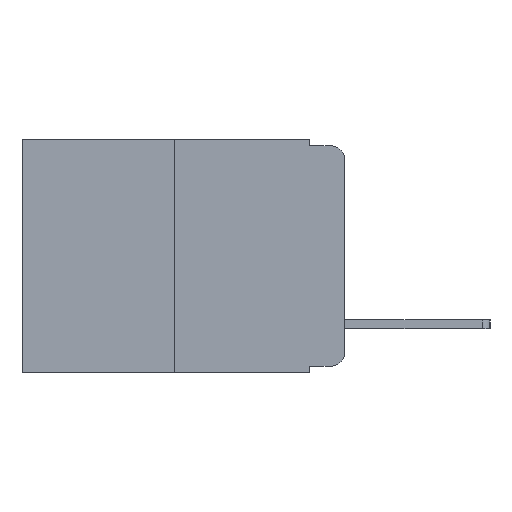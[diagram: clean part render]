
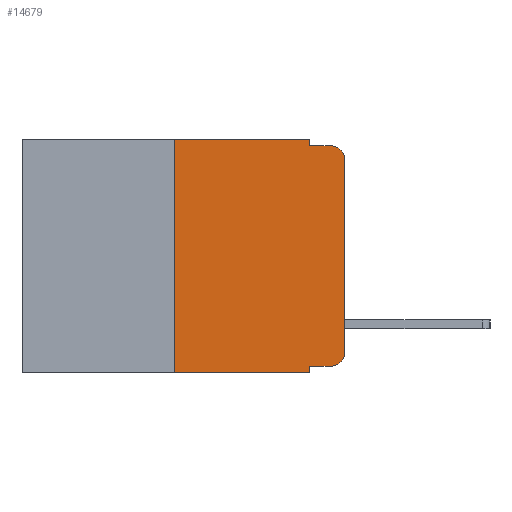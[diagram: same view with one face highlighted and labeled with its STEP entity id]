
A CAD part, left-side view. The second image highlights one B-rep face of the part: STEP entity #14679.
In plain terms, the highlighted planar face has unit normal (-1, 0, 0).
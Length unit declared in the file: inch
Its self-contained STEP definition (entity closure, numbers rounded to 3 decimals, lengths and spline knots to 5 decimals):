
#85 = EDGE_CURVE ( 'NONE', #4995, #4182, #15944, .T. ) ;
#352 = CARTESIAN_POINT ( 'NONE',  ( 0., 0.25, 0. ) ) ;
#551 = VERTEX_POINT ( 'NONE', #2839 ) ;
#724 = CARTESIAN_POINT ( 'NONE',  ( 0., 0., 0. ) ) ;
#828 = EDGE_CURVE ( 'NONE', #551, #3973, #16782, .T. ) ;
#1203 = CARTESIAN_POINT ( 'NONE',  ( 0., 0.02, -0.03 ) ) ;
#1245 = EDGE_CURVE ( 'NONE', #3353, #13988, #9838, .T. ) ;
#1273 = ORIENTED_EDGE ( 'NONE', *, *, #11226, .F. ) ;
#1449 = ORIENTED_EDGE ( 'NONE', *, *, #85, .F. ) ;
#1458 = CARTESIAN_POINT ( 'NONE',  ( 0., 0.051, 0. ) ) ;
#1520 = ORIENTED_EDGE ( 'NONE', *, *, #7905, .F. ) ;
#1824 = LINE ( 'NONE', #1458, #16577 ) ;
#1931 = ORIENTED_EDGE ( 'NONE', *, *, #5646, .F. ) ;
#1948 = LINE ( 'NONE', #6127, #6084 ) ;
#1968 = CARTESIAN_POINT ( 'NONE',  ( 0., 0.051, -0.343 ) ) ;
#2094 = EDGE_CURVE ( 'NONE', #3348, #9759, #4688, .T. ) ;
#2463 = ORIENTED_EDGE ( 'NONE', *, *, #1245, .T. ) ;
#2617 = FACE_OUTER_BOUND ( 'NONE', #7419, .T. ) ;
#2772 = DIRECTION ( 'NONE',  ( -1., 0., 0. ) ) ;
#2788 = DIRECTION ( 'NONE',  ( 0., 0., -1. ) ) ;
#2839 = CARTESIAN_POINT ( 'NONE',  ( 0., 0.25, -0.343 ) ) ;
#3010 = DIRECTION ( 'NONE',  ( 0., -1., 0. ) ) ;
#3069 = DIRECTION ( 'NONE',  ( 0., 0., -1. ) ) ;
#3348 = VERTEX_POINT ( 'NONE', #4824 ) ;
#3353 = VERTEX_POINT ( 'NONE', #8092 ) ;
#3696 = CARTESIAN_POINT ( 'NONE',  ( 0., 0.051, -0.01 ) ) ;
#3754 = AXIS2_PLACEMENT_3D ( 'NONE', #1203, #11410, #2788 ) ;
#3973 = VERTEX_POINT ( 'NONE', #1968 ) ;
#4058 = CARTESIAN_POINT ( 'NONE',  ( 0., 0.02, -0.01 ) ) ;
#4152 = VECTOR ( 'NONE', #7867, 39.37008 ) ;
#4182 = VERTEX_POINT ( 'NONE', #10726 ) ;
#4688 = LINE ( 'NONE', #10905, #15867 ) ;
#4775 = CIRCLE ( 'NONE', #3754, 0.02 ) ;
#4824 = CARTESIAN_POINT ( 'NONE',  ( 0., 0.051, -0.333 ) ) ;
#4995 = VERTEX_POINT ( 'NONE', #352 ) ;
#5646 = EDGE_CURVE ( 'NONE', #551, #4995, #8112, .T. ) ;
#5721 = VECTOR ( 'NONE', #15329, 39.37008 ) ;
#6084 = VECTOR ( 'NONE', #14454, 39.37008 ) ;
#6127 = CARTESIAN_POINT ( 'NONE',  ( 0., 0.051, -0.01 ) ) ;
#6399 = ORIENTED_EDGE ( 'NONE', *, *, #7765, .F. ) ;
#6682 = ORIENTED_EDGE ( 'NONE', *, *, #11048, .T. ) ;
#7239 = VERTEX_POINT ( 'NONE', #3696 ) ;
#7385 = ORIENTED_EDGE ( 'NONE', *, *, #2094, .T. ) ;
#7419 = EDGE_LOOP ( 'NONE', ( #2463, #6682, #6399, #1520, #1449, #1931, #14192, #1273, #7385, #9069 ) ) ;
#7765 = EDGE_CURVE ( 'NONE', #7239, #11688, #1948, .T. ) ;
#7867 = DIRECTION ( 'NONE',  ( 0., 0., -1. ) ) ;
#7905 = EDGE_CURVE ( 'NONE', #4182, #7239, #15404, .T. ) ;
#8092 = CARTESIAN_POINT ( 'NONE',  ( 0., 0., -0.313 ) ) ;
#8112 = LINE ( 'NONE', #16013, #11733 ) ;
#8913 = DIRECTION ( 'NONE',  ( 1., 0., 0. ) ) ;
#9069 = ORIENTED_EDGE ( 'NONE', *, *, #11787, .T. ) ;
#9132 = DIRECTION ( 'NONE',  ( 0., 0., 1. ) ) ;
#9229 = AXIS2_PLACEMENT_3D ( 'NONE', #11644, #8913, #14422 ) ;
#9608 = DIRECTION ( 'NONE',  ( 0., 0., 1. ) ) ;
#9759 = VERTEX_POINT ( 'NONE', #10964 ) ;
#9838 = LINE ( 'NONE', #724, #16767 ) ;
#10294 = DIRECTION ( 'NONE',  ( 0., -1., 0. ) ) ;
#10526 = CARTESIAN_POINT ( 'NONE',  ( 0., 0.473, -0.343 ) ) ;
#10726 = CARTESIAN_POINT ( 'NONE',  ( 0., 0.051, 0. ) ) ;
#10905 = CARTESIAN_POINT ( 'NONE',  ( 0., 0.051, -0.333 ) ) ;
#10964 = CARTESIAN_POINT ( 'NONE',  ( 0., 0.02, -0.333 ) ) ;
#11048 = EDGE_CURVE ( 'NONE', #13988, #11688, #4775, .T. ) ;
#11142 = CARTESIAN_POINT ( 'NONE',  ( 0., 0., -0.03 ) ) ;
#11226 = EDGE_CURVE ( 'NONE', #3348, #3973, #1824, .T. ) ;
#11387 = CARTESIAN_POINT ( 'NONE',  ( 0., 0.02, -0.313 ) ) ;
#11410 = DIRECTION ( 'NONE',  ( -1., 0., 0. ) ) ;
#11644 = CARTESIAN_POINT ( 'NONE',  ( 0., 0.473, 0. ) ) ;
#11688 = VERTEX_POINT ( 'NONE', #4058 ) ;
#11733 = VECTOR ( 'NONE', #9132, 39.37008 ) ;
#11787 = EDGE_CURVE ( 'NONE', #9759, #3353, #12451, .T. ) ;
#12451 = CIRCLE ( 'NONE', #15467, 0.02 ) ;
#12807 = DIRECTION ( 'NONE',  ( 0., 0., -1. ) ) ;
#13040 = PLANE ( 'NONE',  #9229 ) ;
#13988 = VERTEX_POINT ( 'NONE', #11142 ) ;
#14192 = ORIENTED_EDGE ( 'NONE', *, *, #828, .T. ) ;
#14422 = DIRECTION ( 'NONE',  ( 0., 0., -1. ) ) ;
#14454 = DIRECTION ( 'NONE',  ( 0., -1., 0. ) ) ;
#14679 = ADVANCED_FACE ( 'NONE', ( #2617 ), #13040, .F. ) ;
#15329 = DIRECTION ( 'NONE',  ( 0., -1., 0. ) ) ;
#15404 = LINE ( 'NONE', #16104, #4152 ) ;
#15467 = AXIS2_PLACEMENT_3D ( 'NONE', #11387, #2772, #12807 ) ;
#15527 = VECTOR ( 'NONE', #10294, 39.37008 ) ;
#15867 = VECTOR ( 'NONE', #3010, 39.37008 ) ;
#15944 = LINE ( 'NONE', #17191, #15527 ) ;
#16013 = CARTESIAN_POINT ( 'NONE',  ( 0., 0.25, 0. ) ) ;
#16104 = CARTESIAN_POINT ( 'NONE',  ( 0., 0.051, 0. ) ) ;
#16577 = VECTOR ( 'NONE', #3069, 39.37008 ) ;
#16767 = VECTOR ( 'NONE', #9608, 39.37008 ) ;
#16782 = LINE ( 'NONE', #10526, #5721 ) ;
#17191 = CARTESIAN_POINT ( 'NONE',  ( 0., 0.473, 0. ) ) ;
